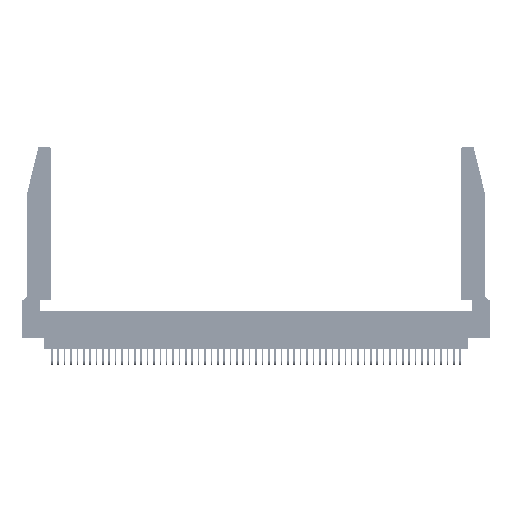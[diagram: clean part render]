
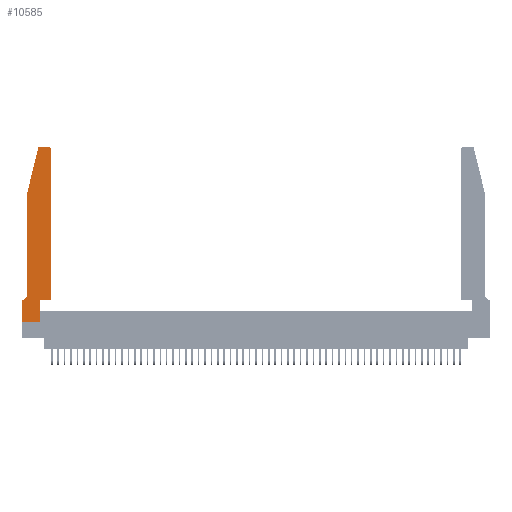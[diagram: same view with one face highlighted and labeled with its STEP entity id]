
A CAD part, top view. The second image highlights one B-rep face of the part: STEP entity #10585.
In plain terms, the highlighted planar face has unit normal (0, 0, 1).
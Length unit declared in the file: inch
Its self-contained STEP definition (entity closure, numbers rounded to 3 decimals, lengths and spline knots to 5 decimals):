
#409 = DIRECTION ( 'NONE',  ( -1., 0., 0. ) ) ;
#452 = LINE ( 'NONE', #24606, #21718 ) ;
#904 = LINE ( 'NONE', #12096, #22140 ) ;
#1343 = VECTOR ( 'NONE', #49380, 39.37008 ) ;
#2034 = AXIS2_PLACEMENT_3D ( 'NONE', #10812, #40331, #15097 ) ;
#2313 = CIRCLE ( 'NONE', #2034, 0.03 ) ;
#4947 = LINE ( 'NONE', #20211, #48357 ) ;
#6032 = CARTESIAN_POINT ( 'NONE',  ( 0.2865, 0., 0.37 ) ) ;
#6309 = CARTESIAN_POINT ( 'NONE',  ( 0.4505, 0.35, 0.37 ) ) ;
#6429 = LINE ( 'NONE', #6309, #27609 ) ;
#7043 = CARTESIAN_POINT ( 'NONE',  ( 0.2865, 0.35, 0.37 ) ) ;
#7267 = ORIENTED_EDGE ( 'NONE', *, *, #39291, .T. ) ;
#7393 = VERTEX_POINT ( 'NONE', #19877 ) ;
#8126 = EDGE_CURVE ( 'NONE', #12279, #7393, #8513, .T. ) ;
#8513 = LINE ( 'NONE', #7043, #29699 ) ;
#8614 = ORIENTED_EDGE ( 'NONE', *, *, #16480, .T. ) ;
#9365 = ORIENTED_EDGE ( 'NONE', *, *, #8126, .T. ) ;
#9990 = ORIENTED_EDGE ( 'NONE', *, *, #17446, .T. ) ;
#10139 = VERTEX_POINT ( 'NONE', #53443 ) ;
#10585 = ADVANCED_FACE ( 'NONE', ( #17487 ), #39610, .T. ) ;
#10812 = CARTESIAN_POINT ( 'NONE',  ( 0.284, 2.72, 0.37 ) ) ;
#12061 = EDGE_CURVE ( 'NONE', #14348, #42105, #43026, .T. ) ;
#12096 = CARTESIAN_POINT ( 'NONE',  ( 0.2605, 2.75, 0.37 ) ) ;
#12157 = ORIENTED_EDGE ( 'NONE', *, *, #36045, .T. ) ;
#12279 = VERTEX_POINT ( 'NONE', #6032 ) ;
#12388 = EDGE_CURVE ( 'NONE', #53814, #31698, #25229, .T. ) ;
#12608 = CARTESIAN_POINT ( 'NONE',  ( 0.0055, 0.35, 0.37 ) ) ;
#13618 = AXIS2_PLACEMENT_3D ( 'NONE', #13706, #43155, #17982 ) ;
#13706 = CARTESIAN_POINT ( 'NONE',  ( 0.4205, 2.72, 0.37 ) ) ;
#14248 = LINE ( 'NONE', #22458, #35350 ) ;
#14338 = VERTEX_POINT ( 'NONE', #34055 ) ;
#14348 = VERTEX_POINT ( 'NONE', #42454 ) ;
#14378 = CARTESIAN_POINT ( 'NONE',  ( 0., 0.35, 0.37 ) ) ;
#15097 = DIRECTION ( 'NONE',  ( 1., 0., 0. ) ) ;
#16113 = ORIENTED_EDGE ( 'NONE', *, *, #27310, .T. ) ;
#16375 = DIRECTION ( 'NONE',  ( -1., 0., 0. ) ) ;
#16480 = EDGE_CURVE ( 'NONE', #42105, #26808, #14248, .T. ) ;
#17446 = EDGE_CURVE ( 'NONE', #26808, #38901, #36554, .T. ) ;
#17487 = FACE_OUTER_BOUND ( 'NONE', #46965, .T. ) ;
#17982 = DIRECTION ( 'NONE',  ( 1., 0., 0. ) ) ;
#18660 = DIRECTION ( 'NONE',  ( 0., 0., 1. ) ) ;
#19003 = CARTESIAN_POINT ( 'NONE',  ( 0.284, 2.75, 0.37 ) ) ;
#19877 = CARTESIAN_POINT ( 'NONE',  ( 0.2865, 0.35, 0.37 ) ) ;
#20211 = CARTESIAN_POINT ( 'NONE',  ( 0., 0., 0.37 ) ) ;
#21341 = CARTESIAN_POINT ( 'NONE',  ( 0., 0., 0.37 ) ) ;
#21718 = VECTOR ( 'NONE', #49634, 39.37008 ) ;
#22140 = VECTOR ( 'NONE', #16375, 39.37008 ) ;
#22458 = CARTESIAN_POINT ( 'NONE',  ( 0.0755, 0.35, 0.37 ) ) ;
#24606 = CARTESIAN_POINT ( 'NONE',  ( 0.0755, 2., 0.37 ) ) ;
#24676 = CARTESIAN_POINT ( 'NONE',  ( 0.4505, 0.35, 0.37 ) ) ;
#25229 = LINE ( 'NONE', #36827, #1343 ) ;
#25844 = DIRECTION ( 'NONE',  ( 0., 0., -1. ) ) ;
#26808 = VERTEX_POINT ( 'NONE', #36216 ) ;
#27310 = EDGE_CURVE ( 'NONE', #10139, #40032, #6429, .T. ) ;
#27609 = VECTOR ( 'NONE', #31604, 39.37008 ) ;
#27964 = CARTESIAN_POINT ( 'NONE',  ( 0.25487, 2.72718, 0.37 ) ) ;
#28128 = DIRECTION ( 'NONE',  ( 0., 1., 0. ) ) ;
#28920 = DIRECTION ( 'NONE',  ( 1., 0., 0. ) ) ;
#29699 = VECTOR ( 'NONE', #28128, 39.37008 ) ;
#30951 = DIRECTION ( 'NONE',  ( -1., 0., 0. ) ) ;
#31326 = VERTEX_POINT ( 'NONE', #19003 ) ;
#31604 = DIRECTION ( 'NONE',  ( 0., 1., 0. ) ) ;
#31698 = VERTEX_POINT ( 'NONE', #44750 ) ;
#32890 = DIRECTION ( 'NONE',  ( 1., 0., 0. ) ) ;
#33056 = ORIENTED_EDGE ( 'NONE', *, *, #52733, .T. ) ;
#33936 = VECTOR ( 'NONE', #49060, 39.37008 ) ;
#34055 = CARTESIAN_POINT ( 'NONE',  ( 0.4205, 2.75, 0.37 ) ) ;
#35350 = VECTOR ( 'NONE', #30951, 39.37008 ) ;
#36045 = EDGE_CURVE ( 'NONE', #31698, #14348, #452, .T. ) ;
#36216 = CARTESIAN_POINT ( 'NONE',  ( 0., 0.35, 0.37 ) ) ;
#36554 = LINE ( 'NONE', #44873, #33936 ) ;
#36827 = CARTESIAN_POINT ( 'NONE',  ( 0.0755, 2., 0.37 ) ) ;
#38901 = VERTEX_POINT ( 'NONE', #21341 ) ;
#39037 = EDGE_CURVE ( 'NONE', #40032, #14338, #41911, .T. ) ;
#39291 = EDGE_CURVE ( 'NONE', #38901, #12279, #4947, .T. ) ;
#39372 = VECTOR ( 'NONE', #28920, 39.37008 ) ;
#39610 = PLANE ( 'NONE',  #44128 ) ;
#40032 = VERTEX_POINT ( 'NONE', #53946 ) ;
#40331 = DIRECTION ( 'NONE',  ( 0., 0., 1. ) ) ;
#40752 = ORIENTED_EDGE ( 'NONE', *, *, #47966, .T. ) ;
#41053 = ORIENTED_EDGE ( 'NONE', *, *, #39037, .T. ) ;
#41911 = CIRCLE ( 'NONE', #13618, 0.03 ) ;
#42105 = VERTEX_POINT ( 'NONE', #12608 ) ;
#42454 = CARTESIAN_POINT ( 'NONE',  ( 0.0755, 0.42, 0.37 ) ) ;
#43026 = CIRCLE ( 'NONE', #48342, 0.07 ) ;
#43155 = DIRECTION ( 'NONE',  ( 0., 0., 1. ) ) ;
#44128 = AXIS2_PLACEMENT_3D ( 'NONE', #14378, #18660, #47967 ) ;
#44750 = CARTESIAN_POINT ( 'NONE',  ( 0.0755, 2., 0.37 ) ) ;
#44873 = CARTESIAN_POINT ( 'NONE',  ( 0., 0., 0.37 ) ) ;
#46080 = ORIENTED_EDGE ( 'NONE', *, *, #12388, .T. ) ;
#46965 = EDGE_LOOP ( 'NONE', ( #40752, #33056, #46080, #12157, #48980, #8614, #9990, #7267, #9365, #49078, #16113, #41053 ) ) ;
#47966 = EDGE_CURVE ( 'NONE', #14338, #31326, #904, .T. ) ;
#47967 = DIRECTION ( 'NONE',  ( 1., 0., 0. ) ) ;
#48342 = AXIS2_PLACEMENT_3D ( 'NONE', #50854, #25844, #409 ) ;
#48357 = VECTOR ( 'NONE', #32890, 39.37008 ) ;
#48980 = ORIENTED_EDGE ( 'NONE', *, *, #12061, .T. ) ;
#49060 = DIRECTION ( 'NONE',  ( 0., -1., 0. ) ) ;
#49078 = ORIENTED_EDGE ( 'NONE', *, *, #51972, .T. ) ;
#49126 = LINE ( 'NONE', #24676, #39372 ) ;
#49380 = DIRECTION ( 'NONE',  ( -0.239, -0.971, 0. ) ) ;
#49634 = DIRECTION ( 'NONE',  ( 0., -1., 0. ) ) ;
#50854 = CARTESIAN_POINT ( 'NONE',  ( 0.0055, 0.42, 0.37 ) ) ;
#51972 = EDGE_CURVE ( 'NONE', #7393, #10139, #49126, .T. ) ;
#52733 = EDGE_CURVE ( 'NONE', #31326, #53814, #2313, .T. ) ;
#53443 = CARTESIAN_POINT ( 'NONE',  ( 0.4505, 0.35, 0.37 ) ) ;
#53814 = VERTEX_POINT ( 'NONE', #27964 ) ;
#53946 = CARTESIAN_POINT ( 'NONE',  ( 0.4505, 2.72, 0.37 ) ) ;
